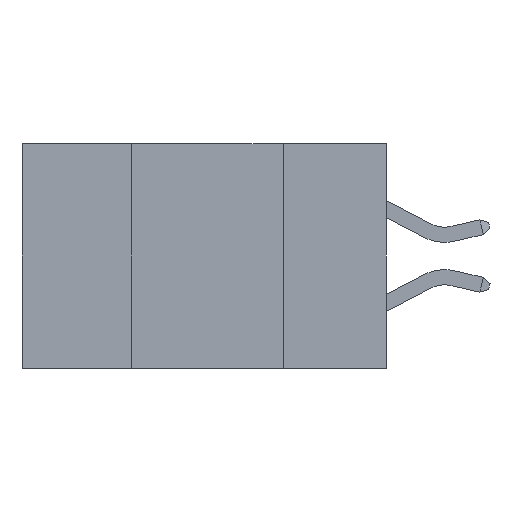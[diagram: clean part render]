
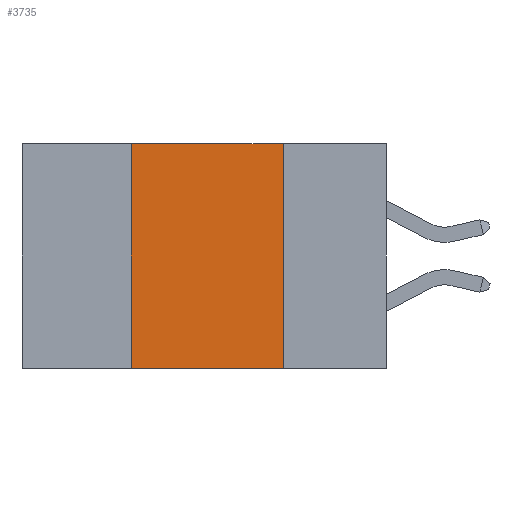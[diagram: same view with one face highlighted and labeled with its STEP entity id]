
A CAD part, left-side view. The second image highlights one B-rep face of the part: STEP entity #3735.
In plain terms, the highlighted planar face has unit normal (-1, 0, 0).
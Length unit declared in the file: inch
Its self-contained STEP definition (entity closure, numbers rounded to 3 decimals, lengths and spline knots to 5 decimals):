
#100 = EDGE_CURVE ( 'NONE', #123, #2713, #7074, .T. ) ;
#123 = VERTEX_POINT ( 'NONE', #7216 ) ;
#306 = EDGE_CURVE ( 'NONE', #2713, #2923, #5125, .T. ) ;
#510 = VECTOR ( 'NONE', #6815, 39.37008 ) ;
#641 = FACE_OUTER_BOUND ( 'NONE', #7950, .T. ) ;
#793 = EDGE_CURVE ( 'NONE', #5690, #2923, #3542, .T. ) ;
#806 = EDGE_CURVE ( 'NONE', #5690, #123, #8519, .T. ) ;
#987 = VECTOR ( 'NONE', #1153, 39.37008 ) ;
#1153 = DIRECTION ( 'NONE',  ( 0., -1., 0. ) ) ;
#1447 = CARTESIAN_POINT ( 'NONE',  ( 0., 0.6, 0. ) ) ;
#1584 = DIRECTION ( 'NONE',  ( 0., 0., 1. ) ) ;
#1741 = CARTESIAN_POINT ( 'NONE',  ( 0., 0.17, -0.37 ) ) ;
#2350 = DIRECTION ( 'NONE',  ( 0., 0., -1. ) ) ;
#2369 = DIRECTION ( 'NONE',  ( 1., 0., 0. ) ) ;
#2484 = PLANE ( 'NONE',  #4739 ) ;
#2633 = CARTESIAN_POINT ( 'NONE',  ( 0., 0.6, 0. ) ) ;
#2713 = VERTEX_POINT ( 'NONE', #8648 ) ;
#2923 = VERTEX_POINT ( 'NONE', #1741 ) ;
#3235 = VECTOR ( 'NONE', #4171, 39.37008 ) ;
#3542 = LINE ( 'NONE', #7796, #3235 ) ;
#3735 = ADVANCED_FACE ( 'NONE', ( #641 ), #2484, .F. ) ;
#4028 = CARTESIAN_POINT ( 'NONE',  ( 0., 0.42, -0.37 ) ) ;
#4171 = DIRECTION ( 'NONE',  ( 0., -1., 0. ) ) ;
#4739 = AXIS2_PLACEMENT_3D ( 'NONE', #2633, #2369, #2350 ) ;
#5125 = LINE ( 'NONE', #6200, #510 ) ;
#5615 = ORIENTED_EDGE ( 'NONE', *, *, #100, .F. ) ;
#5658 = ORIENTED_EDGE ( 'NONE', *, *, #306, .F. ) ;
#5690 = VERTEX_POINT ( 'NONE', #4028 ) ;
#6000 = ORIENTED_EDGE ( 'NONE', *, *, #793, .T. ) ;
#6028 = ORIENTED_EDGE ( 'NONE', *, *, #806, .F. ) ;
#6200 = CARTESIAN_POINT ( 'NONE',  ( 0., 0.17, -0.37 ) ) ;
#6815 = DIRECTION ( 'NONE',  ( 0., 0., -1. ) ) ;
#7074 = LINE ( 'NONE', #1447, #987 ) ;
#7216 = CARTESIAN_POINT ( 'NONE',  ( 0., 0.42, 0. ) ) ;
#7796 = CARTESIAN_POINT ( 'NONE',  ( 0., 0.6, -0.37 ) ) ;
#7950 = EDGE_LOOP ( 'NONE', ( #5658, #5615, #6028, #6000 ) ) ;
#8330 = VECTOR ( 'NONE', #1584, 39.37008 ) ;
#8480 = CARTESIAN_POINT ( 'NONE',  ( 0., 0.42, -0.37 ) ) ;
#8519 = LINE ( 'NONE', #8480, #8330 ) ;
#8648 = CARTESIAN_POINT ( 'NONE',  ( 0., 0.17, 0. ) ) ;
